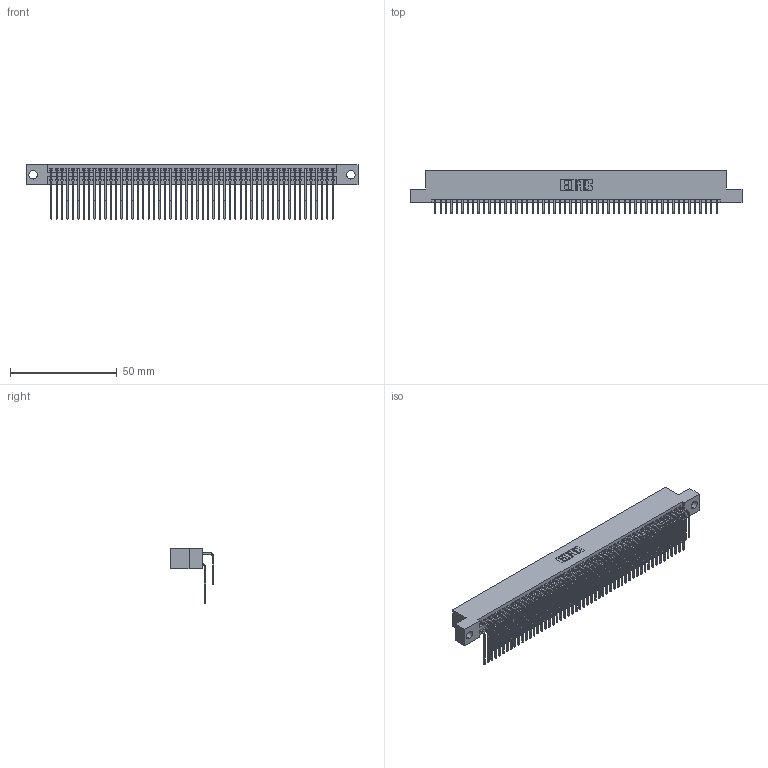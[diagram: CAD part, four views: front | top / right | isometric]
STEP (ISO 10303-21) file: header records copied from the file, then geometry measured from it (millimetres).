
FILE_DESCRIPTION (( 'STEP AP203' ), '1' );
FILE_NAME ('395-106-559-204.STEP', '2018-11-30T18:59:19', ( '' ), ( '' ), 'SwSTEP 2.0', 'SolidWorks 2016', '' );
FILE_SCHEMA (( 'CONFIG_CONTROL_DESIGN' ));
Length unit declared in the file: inch
Products named in the file (4): 345-292-001_558 559 Tail - 1; 345 Part_Flush Mounting Lugs - 0.156 Dia-TH; 345-292-001_559 Tail - 2; 395-106-559-204
Assembly tree (107 placements, depth 2):
  395-106-559-204
    345 Part_Flush Mounting Lugs - 0.156 Dia-TH
    345-292-001_558 559 Tail - 1  x53
    345-292-001_559 Tail - 2  x53
Bounding box: 155.83 x 20.56 x 25.53 mm (x, y, z)
Volume: 15763.1 mm3; surface area: 26204.2 mm2
Topology: 107 solids, 107 shells, 5638 faces, 16771 edges, 11038 vertices
Faces by surface type: plane 3790, cylinder 1848
Entity records: 41759 total; most frequent: CARTESIAN_POINT 7035, ORIENTED_EDGE 6918, DIRECTION 6163, EDGE_CURVE 3459, VECTOR 3075, LINE 3075, VERTEX_POINT 2302, AXIS2_PLACEMENT_3D 1544
